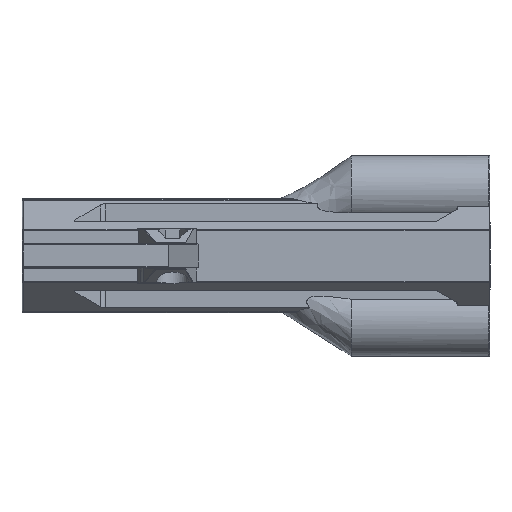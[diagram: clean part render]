
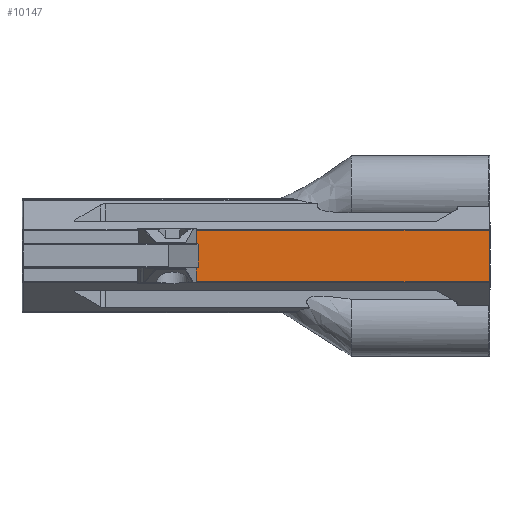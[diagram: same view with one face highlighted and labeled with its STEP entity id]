
A CAD part, front view. The second image highlights one B-rep face of the part: STEP entity #10147.
In plain terms, the highlighted planar face has unit normal (0, -1, 0).
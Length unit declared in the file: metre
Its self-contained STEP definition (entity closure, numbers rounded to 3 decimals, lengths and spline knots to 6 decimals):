
#755=B_SPLINE_CURVE_WITH_KNOTS('',3,(#16161,#16162,#16163,#16164),
 .UNSPECIFIED.,.F.,.F.,(4,4),(0.,0.999892),.UNSPECIFIED.);
#756=B_SPLINE_CURVE_WITH_KNOTS('',3,(#16166,#16167,#16168,#16169),
 .UNSPECIFIED.,.F.,.F.,(4,4),(0.,0.999714),
 .UNSPECIFIED.);
#1647=ORIENTED_EDGE('',*,*,#4641,.F.);
#1648=ORIENTED_EDGE('',*,*,#4642,.T.);
#1649=ORIENTED_EDGE('',*,*,#4643,.T.);
#1650=ORIENTED_EDGE('',*,*,#4644,.T.);
#1651=ORIENTED_EDGE('',*,*,#4645,.T.);
#1652=ORIENTED_EDGE('',*,*,#4646,.T.);
#1653=ORIENTED_EDGE('',*,*,#4647,.T.);
#1654=ORIENTED_EDGE('',*,*,#4648,.T.);
#1655=ORIENTED_EDGE('',*,*,#4649,.T.);
#1656=ORIENTED_EDGE('',*,*,#4650,.F.);
#4641=EDGE_CURVE('',#5697,#6129,#6944,.T.);
#4642=EDGE_CURVE('',#5697,#6130,#755,.T.);
#4643=EDGE_CURVE('',#6130,#6131,#756,.T.);
#4644=EDGE_CURVE('',#6131,#6132,#6945,.T.);
#4645=EDGE_CURVE('',#6132,#6133,#6946,.T.);
#4646=EDGE_CURVE('',#6133,#6134,#6947,.T.);
#4647=EDGE_CURVE('',#6134,#6135,#6948,.T.);
#4648=EDGE_CURVE('',#6135,#6136,#6949,.T.);
#4649=EDGE_CURVE('',#6136,#6137,#6950,.T.);
#4650=EDGE_CURVE('',#6129,#6137,#6951,.T.);
#5697=VERTEX_POINT('',#14238);
#6129=VERTEX_POINT('',#16160);
#6130=VERTEX_POINT('',#16165);
#6131=VERTEX_POINT('',#16170);
#6132=VERTEX_POINT('',#16172);
#6133=VERTEX_POINT('',#16174);
#6134=VERTEX_POINT('',#16176);
#6135=VERTEX_POINT('',#16178);
#6136=VERTEX_POINT('',#16180);
#6137=VERTEX_POINT('',#16182);
#6944=LINE('',#16159,#7844);
#6945=LINE('',#16171,#7845);
#6946=LINE('',#16173,#7846);
#6947=LINE('',#16175,#7847);
#6948=LINE('',#16177,#7848);
#6949=LINE('',#16179,#7849);
#6950=LINE('',#16181,#7850);
#6951=LINE('',#16183,#7851);
#7844=VECTOR('',#12353,1.);
#7845=VECTOR('',#12354,1.);
#7846=VECTOR('',#12355,1.);
#7847=VECTOR('',#12356,1.);
#7848=VECTOR('',#12357,1.);
#7849=VECTOR('',#12358,1.);
#7850=VECTOR('',#12359,1.);
#7851=VECTOR('',#12360,1.);
#8587=EDGE_LOOP('',(#1647,#1648,#1649,#1650,#1651,#1652,#1653,#1654,#1655,
#1656));
#9244=FACE_BOUND('',#8587,.T.);
#9812=PLANE('',#11256);
#10147=ADVANCED_FACE('',(#9244),#9812,.T.);
#11256=AXIS2_PLACEMENT_3D('',#16158,#12351,#12352);
#12351=DIRECTION('',(0.,-1.,0.));
#12352=DIRECTION('',(1.,0.,0.));
#12353=DIRECTION('',(0.,0.,1.));
#12354=DIRECTION('',(1.,0.,0.));
#12355=DIRECTION('',(0.,0.,-1.));
#12356=DIRECTION('',(1.,0.,0.));
#12357=DIRECTION('',(0.,0.,1.));
#12358=DIRECTION('',(-1.,0.,0.));
#12359=DIRECTION('',(0.,0.,-1.));
#12360=DIRECTION('',(1.,0.,0.));
#14238=CARTESIAN_POINT('',(-0.391838,-0.04863,-0.153527));
#16158=CARTESIAN_POINT('',(-0.303847,-0.04863,-0.14773));
#16159=CARTESIAN_POINT('',(-0.391838,-0.04863,-0.14773));
#16160=CARTESIAN_POINT('',(-0.391838,-0.04863,-0.14773));
#16161=CARTESIAN_POINT('',(-0.391838,-0.04863,-0.153527));
#16162=CARTESIAN_POINT('',(-0.391784,-0.04863,-0.153559));
#16163=CARTESIAN_POINT('',(-0.391735,-0.04863,-0.153579));
#16164=CARTESIAN_POINT('',(-0.391683,-0.04863,-0.153579));
#16165=CARTESIAN_POINT('',(-0.391683,-0.048629,-0.153579));
#16166=CARTESIAN_POINT('',(-0.391683,-0.04863,-0.153579));
#16167=CARTESIAN_POINT('',(-0.391683,-0.04863,-0.15412));
#16168=CARTESIAN_POINT('',(-0.391683,-0.04863,-0.15466));
#16169=CARTESIAN_POINT('',(-0.391683,-0.04863,-0.155201));
#16170=CARTESIAN_POINT('',(-0.391683,-0.048629,-0.155201));
#16171=CARTESIAN_POINT('',(-0.303847,-0.04863,-0.155201));
#16172=CARTESIAN_POINT('',(-0.391592,-0.04863,-0.155201));
#16173=CARTESIAN_POINT('',(-0.391592,-0.04863,-0.14773));
#16174=CARTESIAN_POINT('',(-0.391592,-0.04863,-0.159542));
#16175=CARTESIAN_POINT('',(-0.303847,-0.04863,-0.159542));
#16176=CARTESIAN_POINT('',(-0.300049,-0.04863,-0.159542));
#16177=CARTESIAN_POINT('',(-0.300049,-0.04863,-0.143424));
#16178=CARTESIAN_POINT('',(-0.300049,-0.04863,-0.143389));
#16179=CARTESIAN_POINT('',(-0.303847,-0.04863,-0.143389));
#16180=CARTESIAN_POINT('',(-0.391592,-0.04863,-0.143389));
#16181=CARTESIAN_POINT('',(-0.391592,-0.04863,-0.14773));
#16182=CARTESIAN_POINT('',(-0.391592,-0.04863,-0.14773));
#16183=CARTESIAN_POINT('',(-0.391838,-0.04863,-0.14773));
